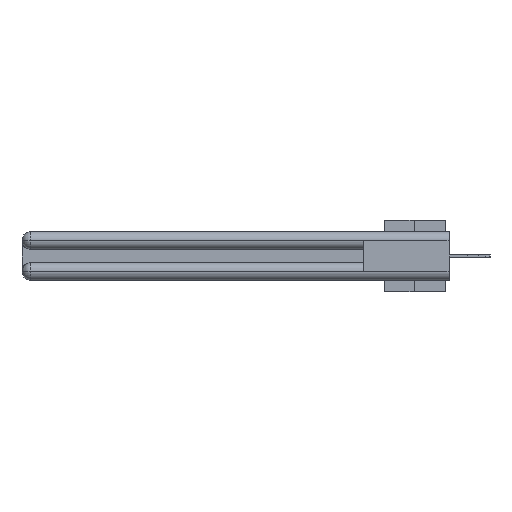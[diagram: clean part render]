
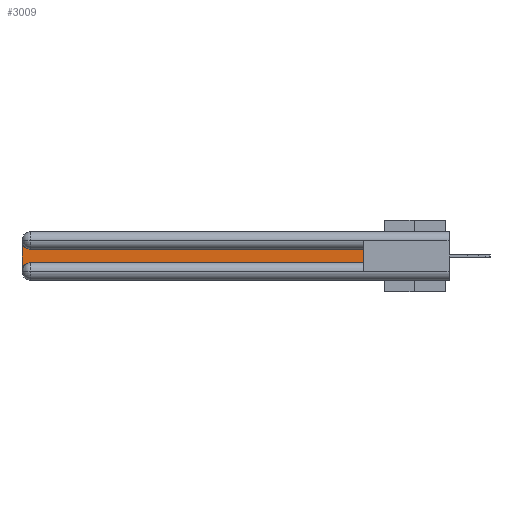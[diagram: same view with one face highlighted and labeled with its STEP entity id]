
A CAD part, left-side view. The second image highlights one B-rep face of the part: STEP entity #3009.
In plain terms, the highlighted planar face has unit normal (-1, 0, 0).
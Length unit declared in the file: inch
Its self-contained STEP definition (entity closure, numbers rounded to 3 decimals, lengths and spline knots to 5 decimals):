
#15 = CARTESIAN_POINT ( 'NONE',  ( 0.075, 2.94, -0.2775 ) ) ;
#194 = EDGE_LOOP ( 'NONE', ( #17464, #2429, #4326, #37067, #30985, #23996 ) ) ;
#1032 = VECTOR ( 'NONE', #9400, 39.37008 ) ;
#1262 = CARTESIAN_POINT ( 'NONE',  ( 0.075, 0.6, -0.2175 ) ) ;
#2138 = CARTESIAN_POINT ( 'NONE',  ( 0.075, 2.94, -0.0625 ) ) ;
#2145 = VECTOR ( 'NONE', #32536, 39.37008 ) ;
#2429 = ORIENTED_EDGE ( 'NONE', *, *, #6015, .T. ) ;
#2937 = EDGE_CURVE ( 'NONE', #24368, #14496, #32677, .T. ) ;
#3009 = ADVANCED_FACE ( 'NONE', ( #15002 ), #12901, .F. ) ;
#3037 = DIRECTION ( 'NONE',  ( 0., 0., -1. ) ) ;
#3081 = LINE ( 'NONE', #5674, #2145 ) ;
#3761 = CARTESIAN_POINT ( 'NONE',  ( 0.075, 3., -0.2775 ) ) ;
#4326 = ORIENTED_EDGE ( 'NONE', *, *, #25169, .T. ) ;
#4879 = CARTESIAN_POINT ( 'NONE',  ( 0.075, 0.6, -0.1225 ) ) ;
#5178 = DIRECTION ( 'NONE',  ( 0., 0., -1. ) ) ;
#5674 = CARTESIAN_POINT ( 'NONE',  ( 0.075, 0.6, -0.2175 ) ) ;
#6015 = EDGE_CURVE ( 'NONE', #13877, #14350, #32295, .T. ) ;
#7016 = DIRECTION ( 'NONE',  ( 1., 0., 0. ) ) ;
#8916 = VECTOR ( 'NONE', #24605, 39.37008 ) ;
#9400 = DIRECTION ( 'NONE',  ( 0., 1., 0. ) ) ;
#12901 = PLANE ( 'NONE',  #27589 ) ;
#13877 = VERTEX_POINT ( 'NONE', #16418 ) ;
#14350 = VERTEX_POINT ( 'NONE', #33300 ) ;
#14496 = VERTEX_POINT ( 'NONE', #1262 ) ;
#15002 = FACE_OUTER_BOUND ( 'NONE', #194, .T. ) ;
#15261 = AXIS2_PLACEMENT_3D ( 'NONE', #15, #20976, #3037 ) ;
#15588 = CARTESIAN_POINT ( 'NONE',  ( 0.075, 2.94, -0.2175 ) ) ;
#15899 = EDGE_CURVE ( 'NONE', #14496, #24715, #3081, .T. ) ;
#16418 = CARTESIAN_POINT ( 'NONE',  ( 0.075, 2.94, -0.1225 ) ) ;
#17464 = ORIENTED_EDGE ( 'NONE', *, *, #34197, .T. ) ;
#19634 = DIRECTION ( 'NONE',  ( 0., 0., -1. ) ) ;
#20976 = DIRECTION ( 'NONE',  ( 1., 0., 0. ) ) ;
#23104 = DIRECTION ( 'NONE',  ( 1., 0., 0. ) ) ;
#23996 = ORIENTED_EDGE ( 'NONE', *, *, #15899, .T. ) ;
#24368 = VERTEX_POINT ( 'NONE', #15588 ) ;
#24412 = VERTEX_POINT ( 'NONE', #3761 ) ;
#24605 = DIRECTION ( 'NONE',  ( 0., -1., 0. ) ) ;
#24715 = VERTEX_POINT ( 'NONE', #4879 ) ;
#24914 = LINE ( 'NONE', #36263, #1032 ) ;
#25169 = EDGE_CURVE ( 'NONE', #14350, #24412, #32804, .T. ) ;
#27589 = AXIS2_PLACEMENT_3D ( 'NONE', #36730, #7016, #27834 ) ;
#27834 = DIRECTION ( 'NONE',  ( 0., 0., -1. ) ) ;
#30985 = ORIENTED_EDGE ( 'NONE', *, *, #2937, .T. ) ;
#31481 = CARTESIAN_POINT ( 'NONE',  ( 0.075, 3., -0.2175 ) ) ;
#31571 = CIRCLE ( 'NONE', #15261, 0.06 ) ;
#31870 = VECTOR ( 'NONE', #19634, 39.37008 ) ;
#32295 = CIRCLE ( 'NONE', #37366, 0.06 ) ;
#32536 = DIRECTION ( 'NONE',  ( 0., 0., 1. ) ) ;
#32677 = LINE ( 'NONE', #33447, #8916 ) ;
#32686 = EDGE_CURVE ( 'NONE', #24412, #24368, #31571, .T. ) ;
#32804 = LINE ( 'NONE', #31481, #31870 ) ;
#33300 = CARTESIAN_POINT ( 'NONE',  ( 0.075, 3., -0.0625 ) ) ;
#33447 = CARTESIAN_POINT ( 'NONE',  ( 0.075, 0.6, -0.2175 ) ) ;
#34197 = EDGE_CURVE ( 'NONE', #24715, #13877, #24914, .T. ) ;
#36263 = CARTESIAN_POINT ( 'NONE',  ( 0.075, 0.6, -0.1225 ) ) ;
#36730 = CARTESIAN_POINT ( 'NONE',  ( 0.075, 3., -0.1225 ) ) ;
#37067 = ORIENTED_EDGE ( 'NONE', *, *, #32686, .T. ) ;
#37366 = AXIS2_PLACEMENT_3D ( 'NONE', #2138, #23104, #5178 ) ;
